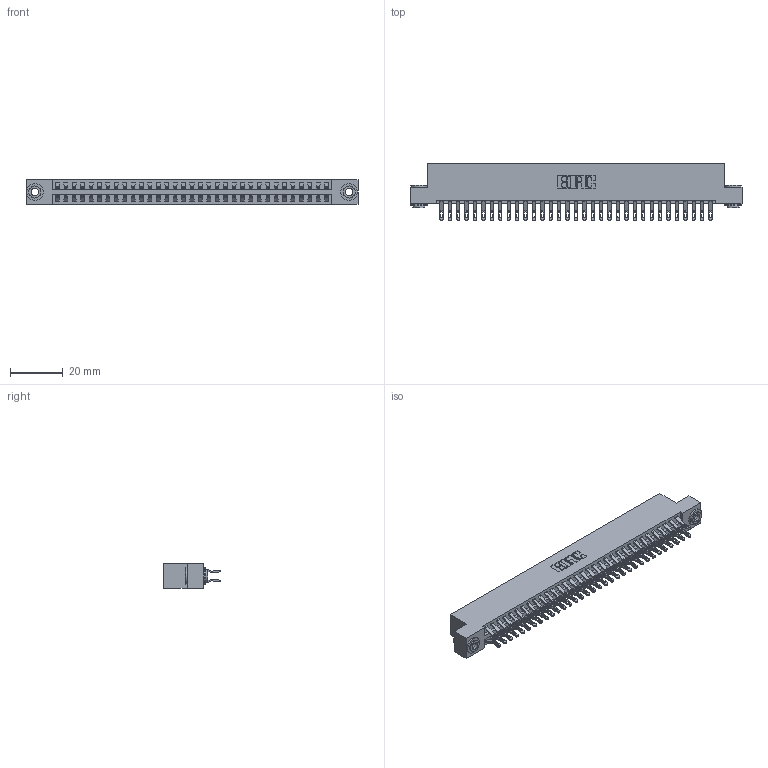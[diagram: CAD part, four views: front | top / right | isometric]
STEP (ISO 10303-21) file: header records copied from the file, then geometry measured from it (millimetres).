
FILE_DESCRIPTION (( 'STEP AP203' ), '1' );
FILE_NAME ('346-066-555-203.STEP', '2018-08-28T11:09:19', ( '' ), ( '' ), 'SwSTEP 2.0', 'SolidWorks 2016', '' );
FILE_SCHEMA (( 'CONFIG_CONTROL_DESIGN' ));
Length unit declared in the file: inch
Products named in the file (4): 346 Part_Flush Mounting Lugs - 0.156 Dia-TH; 345-292-001_555 Tail; 345-250-002_345-250-002-102; 346-066-555-203
Assembly tree (69 placements, depth 2):
  346-066-555-203
    346 Part_Flush Mounting Lugs - 0.156 Dia-TH
    345-292-001_555 Tail  x66
    345-250-002_345-250-002-102  x2
Bounding box: 125.35 x 21.46 x 9.4 mm (x, y, z)
Volume: 12364 mm3; surface area: 17750.3 mm2
Topology: 69 solids, 69 shells, 3988 faces, 12483 edges, 8318 vertices
Faces by surface type: plane 2264, cylinder 1716, cone 8
Entity records: 23724 total; most frequent: CARTESIAN_POINT 3933, ORIENTED_EDGE 3830, DIRECTION 3517, EDGE_CURVE 1915, VECTOR 1607, LINE 1607, VERTEX_POINT 1274, AXIS2_PLACEMENT_3D 955
